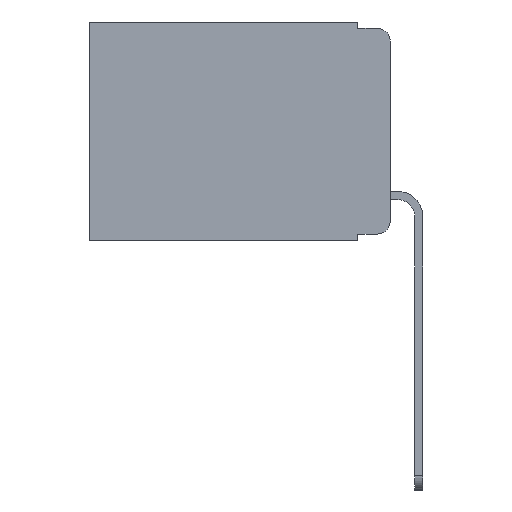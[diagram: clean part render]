
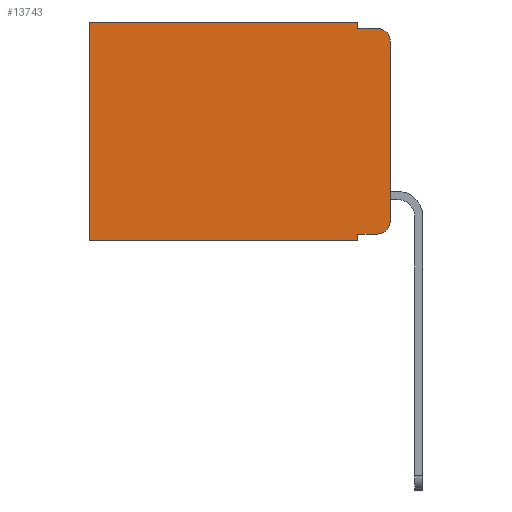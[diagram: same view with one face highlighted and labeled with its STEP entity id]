
A CAD part, left-side view. The second image highlights one B-rep face of the part: STEP entity #13743.
In plain terms, the highlighted planar face has unit normal (-1, 0, 0).
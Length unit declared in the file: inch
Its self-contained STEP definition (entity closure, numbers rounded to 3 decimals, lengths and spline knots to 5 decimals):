
#109 = DIRECTION ( 'NONE',  ( 1., 0., 0. ) ) ;
#1440 = ORIENTED_EDGE ( 'NONE', *, *, #2839, .T. ) ;
#1552 = EDGE_CURVE ( 'NONE', #17321, #15341, #15849, .T. ) ;
#1978 = EDGE_CURVE ( 'NONE', #16493, #10393, #10716, .T. ) ;
#2250 = CARTESIAN_POINT ( 'NONE',  ( 0.298, 0.02, -0.313 ) ) ;
#2330 = VECTOR ( 'NONE', #3082, 39.37008 ) ;
#2839 = EDGE_CURVE ( 'NONE', #16493, #12891, #5349, .T. ) ;
#3082 = DIRECTION ( 'NONE',  ( 0., 0., -1. ) ) ;
#4190 = VERTEX_POINT ( 'NONE', #18158 ) ;
#4517 = EDGE_CURVE ( 'NONE', #10393, #15494, #19497, .T. ) ;
#4792 = CARTESIAN_POINT ( 'NONE',  ( 0.298, 0.051, 0. ) ) ;
#5019 = EDGE_CURVE ( 'NONE', #18067, #14060, #20249, .T. ) ;
#5349 = LINE ( 'NONE', #6080, #20110 ) ;
#5486 = EDGE_CURVE ( 'NONE', #12083, #4190, #12555, .T. ) ;
#5519 = CARTESIAN_POINT ( 'NONE',  ( 0.298, 0.473, -0.343 ) ) ;
#5615 = CARTESIAN_POINT ( 'NONE',  ( 0.298, 0., -0.343 ) ) ;
#5918 = VECTOR ( 'NONE', #14912, 39.37008 ) ;
#6080 = CARTESIAN_POINT ( 'NONE',  ( 0.298, 0.051, -0.333 ) ) ;
#6129 = CARTESIAN_POINT ( 'NONE',  ( 0.298, 0.051, 0. ) ) ;
#6433 = VECTOR ( 'NONE', #7829, 39.37008 ) ;
#6719 = DIRECTION ( 'NONE',  ( 0., -1., 0. ) ) ;
#6994 = VECTOR ( 'NONE', #20287, 39.37008 ) ;
#7829 = DIRECTION ( 'NONE',  ( 0., 0., -1. ) ) ;
#7952 = VECTOR ( 'NONE', #6719, 39.37008 ) ;
#7969 = CARTESIAN_POINT ( 'NONE',  ( 0.298, 0.473, 0. ) ) ;
#8008 = CARTESIAN_POINT ( 'NONE',  ( 0.298, 0.051, -0.333 ) ) ;
#8951 = ORIENTED_EDGE ( 'NONE', *, *, #9777, .T. ) ;
#9777 = EDGE_CURVE ( 'NONE', #17321, #4190, #9786, .T. ) ;
#9786 = CIRCLE ( 'NONE', #18294, 0.02 ) ;
#10271 = ORIENTED_EDGE ( 'NONE', *, *, #4517, .F. ) ;
#10393 = VERTEX_POINT ( 'NONE', #14483 ) ;
#10609 = ORIENTED_EDGE ( 'NONE', *, *, #19425, .F. ) ;
#10716 = LINE ( 'NONE', #6129, #2330 ) ;
#11417 = ORIENTED_EDGE ( 'NONE', *, *, #1552, .F. ) ;
#11512 = LINE ( 'NONE', #7969, #6433 ) ;
#11992 = DIRECTION ( 'NONE',  ( 0., 0., -1. ) ) ;
#12083 = VERTEX_POINT ( 'NONE', #13242 ) ;
#12125 = ORIENTED_EDGE ( 'NONE', *, *, #5019, .T. ) ;
#12226 = AXIS2_PLACEMENT_3D ( 'NONE', #17879, #109, #16415 ) ;
#12555 = LINE ( 'NONE', #16283, #7952 ) ;
#12784 = ORIENTED_EDGE ( 'NONE', *, *, #13579, .T. ) ;
#12891 = VERTEX_POINT ( 'NONE', #15493 ) ;
#13142 = CARTESIAN_POINT ( 'NONE',  ( 0.298, 0.02, -0.03 ) ) ;
#13214 = DIRECTION ( 'NONE',  ( 0., 0., -1. ) ) ;
#13225 = AXIS2_PLACEMENT_3D ( 'NONE', #2250, #18611, #11992 ) ;
#13242 = CARTESIAN_POINT ( 'NONE',  ( 0.298, 0.051, -0.01 ) ) ;
#13579 = EDGE_CURVE ( 'NONE', #14060, #15494, #11512, .T. ) ;
#13626 = CARTESIAN_POINT ( 'NONE',  ( 0.298, 0., 0. ) ) ;
#13743 = ADVANCED_FACE ( 'NONE', ( #19169 ), #16486, .F. ) ;
#14060 = VERTEX_POINT ( 'NONE', #18666 ) ;
#14148 = LINE ( 'NONE', #17579, #17936 ) ;
#14483 = CARTESIAN_POINT ( 'NONE',  ( 0.298, 0.051, -0.343 ) ) ;
#14590 = ORIENTED_EDGE ( 'NONE', *, *, #17047, .T. ) ;
#14641 = DIRECTION ( 'NONE',  ( -1., 0., 0. ) ) ;
#14912 = DIRECTION ( 'NONE',  ( 0., 0., -1. ) ) ;
#15096 = EDGE_LOOP ( 'NONE', ( #11417, #8951, #16731, #10609, #12125, #12784, #10271, #17350, #1440, #14590 ) ) ;
#15341 = VERTEX_POINT ( 'NONE', #21180 ) ;
#15493 = CARTESIAN_POINT ( 'NONE',  ( 0.298, 0.02, -0.333 ) ) ;
#15494 = VERTEX_POINT ( 'NONE', #5519 ) ;
#15580 = CIRCLE ( 'NONE', #13225, 0.02 ) ;
#15653 = DIRECTION ( 'NONE',  ( 0., 1., 0. ) ) ;
#15849 = LINE ( 'NONE', #19492, #5918 ) ;
#16283 = CARTESIAN_POINT ( 'NONE',  ( 0.298, 0.051, -0.01 ) ) ;
#16415 = DIRECTION ( 'NONE',  ( 0., 0., -1. ) ) ;
#16486 = PLANE ( 'NONE',  #12226 ) ;
#16493 = VERTEX_POINT ( 'NONE', #8008 ) ;
#16731 = ORIENTED_EDGE ( 'NONE', *, *, #5486, .F. ) ;
#17047 = EDGE_CURVE ( 'NONE', #12891, #15341, #15580, .T. ) ;
#17321 = VERTEX_POINT ( 'NONE', #17387 ) ;
#17350 = ORIENTED_EDGE ( 'NONE', *, *, #1978, .F. ) ;
#17387 = CARTESIAN_POINT ( 'NONE',  ( 0.298, 0., -0.03 ) ) ;
#17579 = CARTESIAN_POINT ( 'NONE',  ( 0.298, 0.051, 0. ) ) ;
#17879 = CARTESIAN_POINT ( 'NONE',  ( 0.298, 0., 0. ) ) ;
#17936 = VECTOR ( 'NONE', #18145, 39.37008 ) ;
#18067 = VERTEX_POINT ( 'NONE', #4792 ) ;
#18145 = DIRECTION ( 'NONE',  ( 0., 0., -1. ) ) ;
#18158 = CARTESIAN_POINT ( 'NONE',  ( 0.298, 0.02, -0.01 ) ) ;
#18294 = AXIS2_PLACEMENT_3D ( 'NONE', #13142, #14641, #13214 ) ;
#18611 = DIRECTION ( 'NONE',  ( -1., 0., 0. ) ) ;
#18666 = CARTESIAN_POINT ( 'NONE',  ( 0.298, 0.473, 0. ) ) ;
#19169 = FACE_OUTER_BOUND ( 'NONE', #15096, .T. ) ;
#19425 = EDGE_CURVE ( 'NONE', #18067, #12083, #14148, .T. ) ;
#19475 = VECTOR ( 'NONE', #15653, 39.37008 ) ;
#19492 = CARTESIAN_POINT ( 'NONE',  ( 0.298, 0., 0. ) ) ;
#19497 = LINE ( 'NONE', #5615, #6994 ) ;
#20110 = VECTOR ( 'NONE', #20826, 39.37008 ) ;
#20249 = LINE ( 'NONE', #13626, #19475 ) ;
#20287 = DIRECTION ( 'NONE',  ( 0., 1., 0. ) ) ;
#20826 = DIRECTION ( 'NONE',  ( 0., -1., 0. ) ) ;
#21180 = CARTESIAN_POINT ( 'NONE',  ( 0.298, 0., -0.313 ) ) ;
